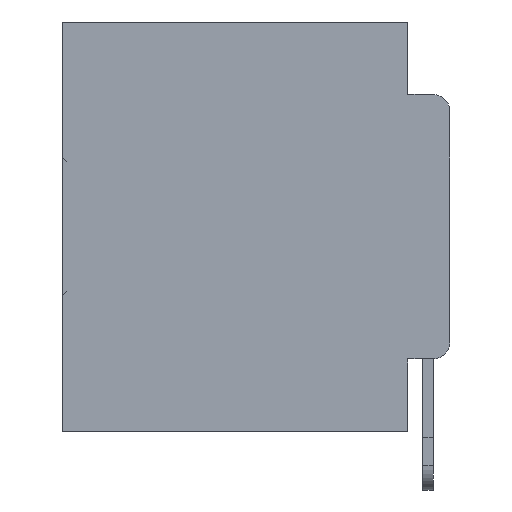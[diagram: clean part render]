
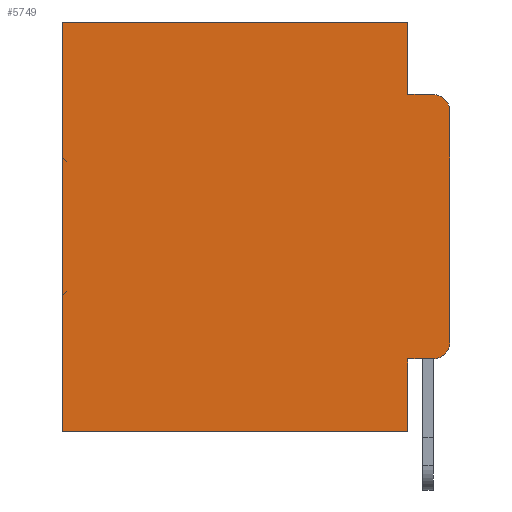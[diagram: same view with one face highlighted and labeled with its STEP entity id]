
A CAD part, left-side view. The second image highlights one B-rep face of the part: STEP entity #5749.
In plain terms, the highlighted planar face has unit normal (-1, 0, 0).
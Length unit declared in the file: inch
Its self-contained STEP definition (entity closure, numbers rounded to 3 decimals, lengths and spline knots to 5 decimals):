
#305 = VERTEX_POINT ( 'NONE', #13883 ) ;
#380 = DIRECTION ( 'NONE',  ( 0., -1., 0. ) ) ;
#775 = EDGE_CURVE ( 'NONE', #28762, #31499, #20405, .T. ) ;
#1177 = ORIENTED_EDGE ( 'NONE', *, *, #7021, .T. ) ;
#2048 = LINE ( 'NONE', #20071, #16081 ) ;
#2848 = VERTEX_POINT ( 'NONE', #9998 ) ;
#2943 = ORIENTED_EDGE ( 'NONE', *, *, #5047, .F. ) ;
#3697 = EDGE_LOOP ( 'NONE', ( #29942, #4289, #31473, #19732, #20518, #1177, #2943, #10053, #31887, #26017 ) ) ;
#4170 = CARTESIAN_POINT ( 'NONE',  ( 0.298, 0.02, -0.0885 ) ) ;
#4289 = ORIENTED_EDGE ( 'NONE', *, *, #22506, .T. ) ;
#4424 = CARTESIAN_POINT ( 'NONE',  ( 0.298, 0.051, -0.0885 ) ) ;
#4535 = DIRECTION ( 'NONE',  ( 0., 0., -1. ) ) ;
#4568 = VECTOR ( 'NONE', #27025, 39.37008 ) ;
#5047 = EDGE_CURVE ( 'NONE', #18302, #305, #32356, .T. ) ;
#5230 = CARTESIAN_POINT ( 'NONE',  ( 0.298, 0.051, 0. ) ) ;
#5261 = EDGE_CURVE ( 'NONE', #31705, #18302, #10938, .T. ) ;
#5749 = ADVANCED_FACE ( 'NONE', ( #25680 ), #26979, .F. ) ;
#6057 = LINE ( 'NONE', #4424, #26478 ) ;
#7021 = EDGE_CURVE ( 'NONE', #2848, #305, #2048, .T. ) ;
#7533 = VECTOR ( 'NONE', #7861, 39.37008 ) ;
#7861 = DIRECTION ( 'NONE',  ( 0., 0., -1. ) ) ;
#8761 = EDGE_CURVE ( 'NONE', #29758, #12119, #15204, .T. ) ;
#9272 = DIRECTION ( 'NONE',  ( 0., 0., -1. ) ) ;
#9998 = CARTESIAN_POINT ( 'NONE',  ( 0.298, 0.473, 0. ) ) ;
#10053 = ORIENTED_EDGE ( 'NONE', *, *, #5261, .F. ) ;
#10938 = LINE ( 'NONE', #32034, #16987 ) ;
#10987 = VERTEX_POINT ( 'NONE', #22474 ) ;
#12119 = VERTEX_POINT ( 'NONE', #28738 ) ;
#13537 = VECTOR ( 'NONE', #13740, 39.37008 ) ;
#13740 = DIRECTION ( 'NONE',  ( 0., 0., -1. ) ) ;
#13883 = CARTESIAN_POINT ( 'NONE',  ( 0.298, 0.473, -0.5 ) ) ;
#14276 = DIRECTION ( 'NONE',  ( 0., 0., -1. ) ) ;
#14633 = CARTESIAN_POINT ( 'NONE',  ( 0.298, 0.02, -0.3915 ) ) ;
#15204 = LINE ( 'NONE', #5230, #7533 ) ;
#15332 = CARTESIAN_POINT ( 'NONE',  ( 0.298, 0.02, -0.1085 ) ) ;
#15833 = CARTESIAN_POINT ( 'NONE',  ( 0.298, 0., -0.5 ) ) ;
#16081 = VECTOR ( 'NONE', #4535, 39.37008 ) ;
#16131 = VERTEX_POINT ( 'NONE', #4170 ) ;
#16839 = CARTESIAN_POINT ( 'NONE',  ( 0.298, 0., 0. ) ) ;
#16987 = VECTOR ( 'NONE', #9272, 39.37008 ) ;
#17269 = DIRECTION ( 'NONE',  ( 0., 0., -1. ) ) ;
#17789 = AXIS2_PLACEMENT_3D ( 'NONE', #24409, #29517, #14276 ) ;
#17981 = DIRECTION ( 'NONE',  ( 0., 0., -1. ) ) ;
#18302 = VERTEX_POINT ( 'NONE', #28445 ) ;
#18416 = LINE ( 'NONE', #16839, #4568 ) ;
#18421 = LINE ( 'NONE', #31416, #30971 ) ;
#18459 = DIRECTION ( 'NONE',  ( 0., 1., 0. ) ) ;
#19042 = VECTOR ( 'NONE', #18459, 39.37008 ) ;
#19171 = EDGE_CURVE ( 'NONE', #12119, #16131, #6057, .T. ) ;
#19732 = ORIENTED_EDGE ( 'NONE', *, *, #8761, .F. ) ;
#20071 = CARTESIAN_POINT ( 'NONE',  ( 0.298, 0.473, 0. ) ) ;
#20405 = LINE ( 'NONE', #26740, #13537 ) ;
#20518 = ORIENTED_EDGE ( 'NONE', *, *, #29173, .T. ) ;
#20818 = CARTESIAN_POINT ( 'NONE',  ( 0.298, 0.051, 0. ) ) ;
#20902 = AXIS2_PLACEMENT_3D ( 'NONE', #15332, #33000, #17981 ) ;
#21460 = EDGE_CURVE ( 'NONE', #10987, #31499, #26632, .T. ) ;
#22470 = DIRECTION ( 'NONE',  ( 0., -1., 0. ) ) ;
#22474 = CARTESIAN_POINT ( 'NONE',  ( 0.298, 0.02, -0.4115 ) ) ;
#22506 = EDGE_CURVE ( 'NONE', #28762, #16131, #30106, .T. ) ;
#24409 = CARTESIAN_POINT ( 'NONE',  ( 0.298, 0., 0. ) ) ;
#25680 = FACE_OUTER_BOUND ( 'NONE', #3697, .T. ) ;
#25884 = CARTESIAN_POINT ( 'NONE',  ( 0.298, 0., -0.3915 ) ) ;
#26017 = ORIENTED_EDGE ( 'NONE', *, *, #21460, .T. ) ;
#26478 = VECTOR ( 'NONE', #22470, 39.37008 ) ;
#26632 = CIRCLE ( 'NONE', #28463, 0.02 ) ;
#26648 = CARTESIAN_POINT ( 'NONE',  ( 0.298, 0.051, -0.4115 ) ) ;
#26740 = CARTESIAN_POINT ( 'NONE',  ( 0.298, 0., 0. ) ) ;
#26979 = PLANE ( 'NONE',  #17789 ) ;
#27025 = DIRECTION ( 'NONE',  ( 0., 1., 0. ) ) ;
#28445 = CARTESIAN_POINT ( 'NONE',  ( 0.298, 0.051, -0.5 ) ) ;
#28463 = AXIS2_PLACEMENT_3D ( 'NONE', #14633, #32319, #17269 ) ;
#28738 = CARTESIAN_POINT ( 'NONE',  ( 0.298, 0.051, -0.0885 ) ) ;
#28762 = VERTEX_POINT ( 'NONE', #30539 ) ;
#29173 = EDGE_CURVE ( 'NONE', #29758, #2848, #18416, .T. ) ;
#29517 = DIRECTION ( 'NONE',  ( 1., 0., 0. ) ) ;
#29758 = VERTEX_POINT ( 'NONE', #20818 ) ;
#29892 = EDGE_CURVE ( 'NONE', #31705, #10987, #18421, .T. ) ;
#29942 = ORIENTED_EDGE ( 'NONE', *, *, #775, .F. ) ;
#30106 = CIRCLE ( 'NONE', #20902, 0.02 ) ;
#30539 = CARTESIAN_POINT ( 'NONE',  ( 0.298, 0., -0.1085 ) ) ;
#30971 = VECTOR ( 'NONE', #380, 39.37008 ) ;
#31416 = CARTESIAN_POINT ( 'NONE',  ( 0.298, 0.051, -0.4115 ) ) ;
#31473 = ORIENTED_EDGE ( 'NONE', *, *, #19171, .F. ) ;
#31499 = VERTEX_POINT ( 'NONE', #25884 ) ;
#31705 = VERTEX_POINT ( 'NONE', #26648 ) ;
#31887 = ORIENTED_EDGE ( 'NONE', *, *, #29892, .T. ) ;
#32034 = CARTESIAN_POINT ( 'NONE',  ( 0.298, 0.051, 0. ) ) ;
#32319 = DIRECTION ( 'NONE',  ( -1., 0., 0. ) ) ;
#32356 = LINE ( 'NONE', #15833, #19042 ) ;
#33000 = DIRECTION ( 'NONE',  ( -1., 0., 0. ) ) ;
